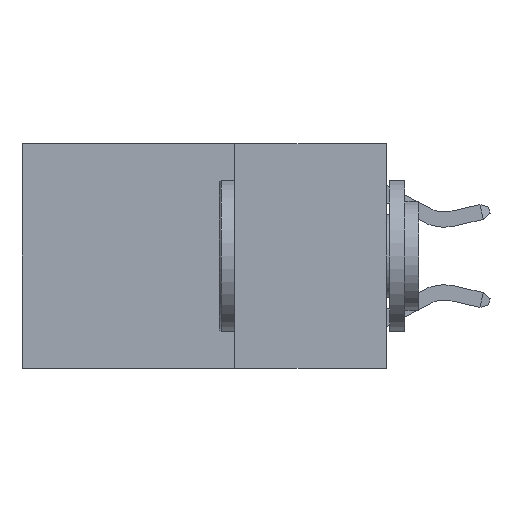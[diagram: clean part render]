
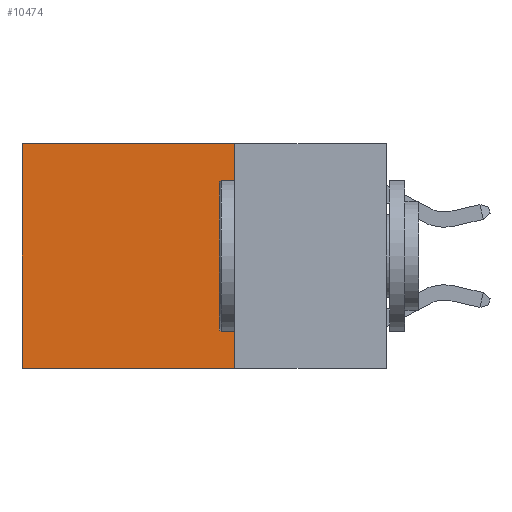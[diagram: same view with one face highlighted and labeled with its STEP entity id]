
A CAD part, left-side view. The second image highlights one B-rep face of the part: STEP entity #10474.
In plain terms, the highlighted planar face has unit normal (-1, 0, 0).
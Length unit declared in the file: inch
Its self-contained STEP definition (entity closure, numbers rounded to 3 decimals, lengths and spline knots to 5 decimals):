
#408 = CARTESIAN_POINT ( 'NONE',  ( 0.2625, 0.6, -0.37 ) ) ;
#703 = CARTESIAN_POINT ( 'NONE',  ( 0.2625, 0.25, -0.37 ) ) ;
#2311 = FACE_OUTER_BOUND ( 'NONE', #14365, .T. ) ;
#2646 = ORIENTED_EDGE ( 'NONE', *, *, #26340, .T. ) ;
#3179 = CARTESIAN_POINT ( 'NONE',  ( 0.2625, 0.6, 0. ) ) ;
#5845 = DIRECTION ( 'NONE',  ( 0., 0., -1. ) ) ;
#6095 = DIRECTION ( 'NONE',  ( 0., 0., -1. ) ) ;
#6551 = VECTOR ( 'NONE', #19972, 39.37008 ) ;
#7411 = VECTOR ( 'NONE', #5845, 39.37008 ) ;
#7769 = AXIS2_PLACEMENT_3D ( 'NONE', #18332, #13885, #6095 ) ;
#8268 = VECTOR ( 'NONE', #10138, 39.37008 ) ;
#10138 = DIRECTION ( 'NONE',  ( 0., 1., 0. ) ) ;
#10474 = ADVANCED_FACE ( 'NONE', ( #2311 ), #26302, .F. ) ;
#10750 = VERTEX_POINT ( 'NONE', #25662 ) ;
#13885 = DIRECTION ( 'NONE',  ( 1., 0., 0. ) ) ;
#14365 = EDGE_LOOP ( 'NONE', ( #2646, #20860, #21708, #25712 ) ) ;
#14790 = EDGE_CURVE ( 'NONE', #10750, #17758, #16073, .T. ) ;
#16073 = LINE ( 'NONE', #22270, #7411 ) ;
#16466 = CARTESIAN_POINT ( 'NONE',  ( 0.2625, 0.25, -0.37 ) ) ;
#17126 = EDGE_CURVE ( 'NONE', #17758, #24271, #22387, .T. ) ;
#17758 = VERTEX_POINT ( 'NONE', #703 ) ;
#18332 = CARTESIAN_POINT ( 'NONE',  ( 0.2625, 0.25, 0. ) ) ;
#19972 = DIRECTION ( 'NONE',  ( 0., 0., -1. ) ) ;
#19992 = VECTOR ( 'NONE', #20324, 39.37008 ) ;
#20057 = CARTESIAN_POINT ( 'NONE',  ( 0.2625, 0.25, 0. ) ) ;
#20324 = DIRECTION ( 'NONE',  ( 0., 1., 0. ) ) ;
#20860 = ORIENTED_EDGE ( 'NONE', *, *, #17126, .F. ) ;
#21708 = ORIENTED_EDGE ( 'NONE', *, *, #14790, .F. ) ;
#21857 = LINE ( 'NONE', #3179, #6551 ) ;
#22270 = CARTESIAN_POINT ( 'NONE',  ( 0.2625, 0.25, 0. ) ) ;
#22387 = LINE ( 'NONE', #16466, #8268 ) ;
#22940 = VERTEX_POINT ( 'NONE', #23089 ) ;
#23089 = CARTESIAN_POINT ( 'NONE',  ( 0.2625, 0.6, 0. ) ) ;
#24271 = VERTEX_POINT ( 'NONE', #408 ) ;
#24642 = LINE ( 'NONE', #20057, #19992 ) ;
#25586 = EDGE_CURVE ( 'NONE', #10750, #22940, #24642, .T. ) ;
#25662 = CARTESIAN_POINT ( 'NONE',  ( 0.2625, 0.25, 0. ) ) ;
#25712 = ORIENTED_EDGE ( 'NONE', *, *, #25586, .T. ) ;
#26302 = PLANE ( 'NONE',  #7769 ) ;
#26340 = EDGE_CURVE ( 'NONE', #22940, #24271, #21857, .T. ) ;
